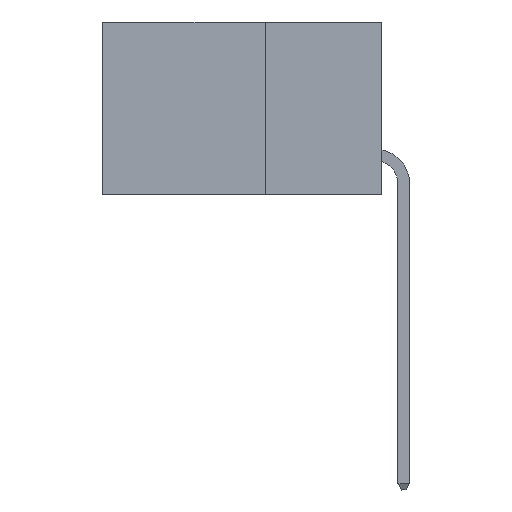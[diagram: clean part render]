
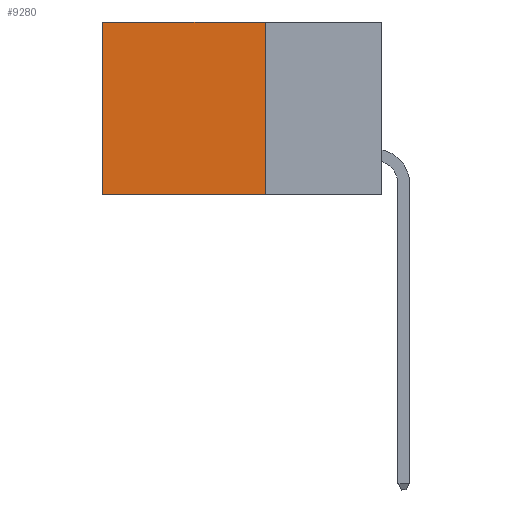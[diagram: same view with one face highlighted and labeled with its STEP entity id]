
A CAD part, left-side view. The second image highlights one B-rep face of the part: STEP entity #9280.
In plain terms, the highlighted planar face has unit normal (-1, 0, 0).
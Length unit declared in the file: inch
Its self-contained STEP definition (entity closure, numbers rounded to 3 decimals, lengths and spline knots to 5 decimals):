
#78 = CARTESIAN_POINT ( 'NONE',  ( 0.2875, 0.6, -0.37 ) ) ;
#2326 = CARTESIAN_POINT ( 'NONE',  ( 0.2875, 0.25, 0. ) ) ;
#2442 = DIRECTION ( 'NONE',  ( 1., 0., 0. ) ) ;
#3063 = VECTOR ( 'NONE', #28266, 39.37008 ) ;
#3181 = ORIENTED_EDGE ( 'NONE', *, *, #30481, .T. ) ;
#4591 = AXIS2_PLACEMENT_3D ( 'NONE', #4838, #2442, #17126 ) ;
#4838 = CARTESIAN_POINT ( 'NONE',  ( 0.2875, 0.25, 0. ) ) ;
#6269 = VECTOR ( 'NONE', #18799, 39.37008 ) ;
#7006 = DIRECTION ( 'NONE',  ( 0., 1., 0. ) ) ;
#7295 = CARTESIAN_POINT ( 'NONE',  ( 0.2875, 0.25, 0. ) ) ;
#7898 = ORIENTED_EDGE ( 'NONE', *, *, #25644, .F. ) ;
#9280 = ADVANCED_FACE ( 'NONE', ( #27009 ), #26680, .F. ) ;
#9393 = ORIENTED_EDGE ( 'NONE', *, *, #16586, .T. ) ;
#11517 = CARTESIAN_POINT ( 'NONE',  ( 0.2875, 0.25, 0. ) ) ;
#11795 = LINE ( 'NONE', #7295, #6269 ) ;
#12253 = VERTEX_POINT ( 'NONE', #30460 ) ;
#13116 = CARTESIAN_POINT ( 'NONE',  ( 0.2875, 0.6, 0. ) ) ;
#13616 = LINE ( 'NONE', #11517, #3063 ) ;
#14033 = VERTEX_POINT ( 'NONE', #2326 ) ;
#15088 = EDGE_CURVE ( 'NONE', #30457, #25404, #17066, .T. ) ;
#15111 = ORIENTED_EDGE ( 'NONE', *, *, #15088, .F. ) ;
#15215 = EDGE_LOOP ( 'NONE', ( #9393, #15111, #7898, #3181 ) ) ;
#15654 = VECTOR ( 'NONE', #18056, 39.37008 ) ;
#16586 = EDGE_CURVE ( 'NONE', #12253, #25404, #18205, .T. ) ;
#17066 = LINE ( 'NONE', #17392, #26999 ) ;
#17126 = DIRECTION ( 'NONE',  ( 0., 0., -1. ) ) ;
#17392 = CARTESIAN_POINT ( 'NONE',  ( 0.2875, 0.25, -0.37 ) ) ;
#18056 = DIRECTION ( 'NONE',  ( 0., 0., -1. ) ) ;
#18205 = LINE ( 'NONE', #13116, #15654 ) ;
#18799 = DIRECTION ( 'NONE',  ( 0., 1., 0. ) ) ;
#21655 = CARTESIAN_POINT ( 'NONE',  ( 0.2875, 0.25, -0.37 ) ) ;
#25404 = VERTEX_POINT ( 'NONE', #78 ) ;
#25644 = EDGE_CURVE ( 'NONE', #14033, #30457, #13616, .T. ) ;
#26680 = PLANE ( 'NONE',  #4591 ) ;
#26999 = VECTOR ( 'NONE', #7006, 39.37008 ) ;
#27009 = FACE_OUTER_BOUND ( 'NONE', #15215, .T. ) ;
#28266 = DIRECTION ( 'NONE',  ( 0., 0., -1. ) ) ;
#30457 = VERTEX_POINT ( 'NONE', #21655 ) ;
#30460 = CARTESIAN_POINT ( 'NONE',  ( 0.2875, 0.6, 0. ) ) ;
#30481 = EDGE_CURVE ( 'NONE', #14033, #12253, #11795, .T. ) ;
